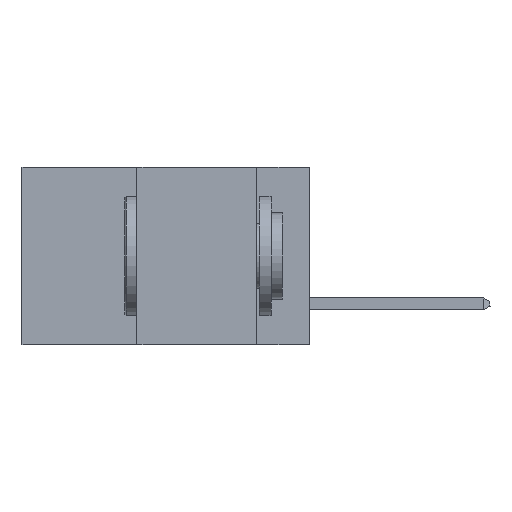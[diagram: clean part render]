
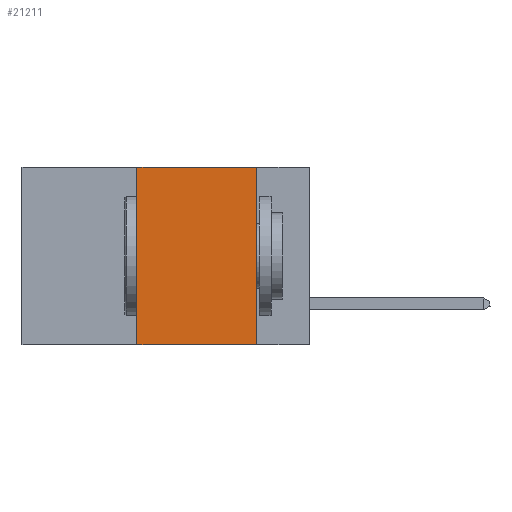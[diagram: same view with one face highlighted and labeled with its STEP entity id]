
A CAD part, left-side view. The second image highlights one B-rep face of the part: STEP entity #21211.
In plain terms, the highlighted planar face has unit normal (-1, 0, 0).
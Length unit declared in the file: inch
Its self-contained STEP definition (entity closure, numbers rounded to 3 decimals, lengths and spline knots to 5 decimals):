
#486 = VECTOR ( 'NONE', #29898, 39.37008 ) ;
#1004 = VECTOR ( 'NONE', #32978, 39.37008 ) ;
#1458 = AXIS2_PLACEMENT_3D ( 'NONE', #14939, #14823, #28697 ) ;
#1653 = ORIENTED_EDGE ( 'NONE', *, *, #14123, .T. ) ;
#3018 = VERTEX_POINT ( 'NONE', #33256 ) ;
#3360 = LINE ( 'NONE', #29096, #17087 ) ;
#5718 = LINE ( 'NONE', #30226, #1004 ) ;
#6614 = EDGE_LOOP ( 'NONE', ( #11829, #28370, #33744, #1653 ) ) ;
#9547 = PLANE ( 'NONE',  #1458 ) ;
#11829 = ORIENTED_EDGE ( 'NONE', *, *, #35378, .F. ) ;
#13668 = VERTEX_POINT ( 'NONE', #17166 ) ;
#14123 = EDGE_CURVE ( 'NONE', #13668, #3018, #5718, .T. ) ;
#14823 = DIRECTION ( 'NONE',  ( 1., 0., 0. ) ) ;
#14939 = CARTESIAN_POINT ( 'NONE',  ( 0., 0.6, 0. ) ) ;
#15274 = EDGE_CURVE ( 'NONE', #13668, #25906, #20587, .T. ) ;
#17087 = VECTOR ( 'NONE', #23190, 39.37008 ) ;
#17166 = CARTESIAN_POINT ( 'NONE',  ( 0., 0.36, -0.37 ) ) ;
#18634 = CARTESIAN_POINT ( 'NONE',  ( 0., 0.36, 0. ) ) ;
#19327 = FACE_OUTER_BOUND ( 'NONE', #6614, .T. ) ;
#20587 = LINE ( 'NONE', #35048, #486 ) ;
#20775 = CARTESIAN_POINT ( 'NONE',  ( 0., 0.11, 0. ) ) ;
#20789 = DIRECTION ( 'NONE',  ( 0., -1., 0. ) ) ;
#21211 = ADVANCED_FACE ( 'NONE', ( #19327 ), #9547, .F. ) ;
#22443 = VECTOR ( 'NONE', #20789, 39.37008 ) ;
#23190 = DIRECTION ( 'NONE',  ( 0., 0., -1. ) ) ;
#25126 = EDGE_CURVE ( 'NONE', #25906, #28982, #29764, .T. ) ;
#25906 = VERTEX_POINT ( 'NONE', #18634 ) ;
#28370 = ORIENTED_EDGE ( 'NONE', *, *, #25126, .F. ) ;
#28697 = DIRECTION ( 'NONE',  ( 0., 0., -1. ) ) ;
#28982 = VERTEX_POINT ( 'NONE', #20775 ) ;
#29069 = CARTESIAN_POINT ( 'NONE',  ( 0., 0.6, 0. ) ) ;
#29096 = CARTESIAN_POINT ( 'NONE',  ( 0., 0.11, 0. ) ) ;
#29764 = LINE ( 'NONE', #29069, #22443 ) ;
#29898 = DIRECTION ( 'NONE',  ( 0., 0., 1. ) ) ;
#30226 = CARTESIAN_POINT ( 'NONE',  ( 0., 0.6, -0.37 ) ) ;
#32978 = DIRECTION ( 'NONE',  ( 0., -1., 0. ) ) ;
#33256 = CARTESIAN_POINT ( 'NONE',  ( 0., 0.11, -0.37 ) ) ;
#33744 = ORIENTED_EDGE ( 'NONE', *, *, #15274, .F. ) ;
#35048 = CARTESIAN_POINT ( 'NONE',  ( 0., 0.36, 0. ) ) ;
#35378 = EDGE_CURVE ( 'NONE', #28982, #3018, #3360, .T. ) ;
